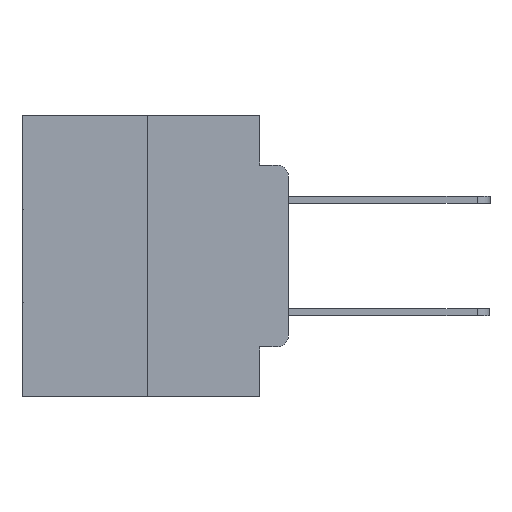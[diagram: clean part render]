
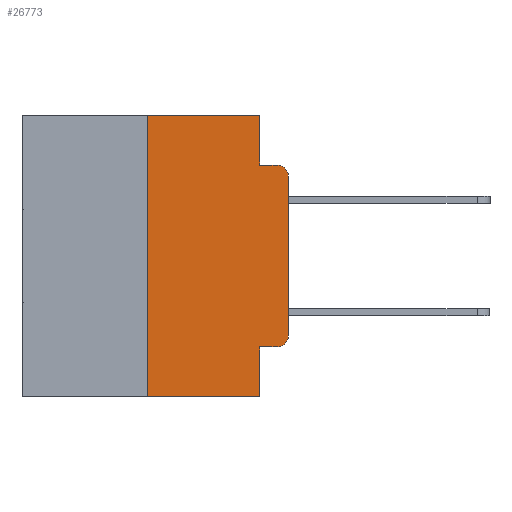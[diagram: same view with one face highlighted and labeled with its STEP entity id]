
A CAD part, left-side view. The second image highlights one B-rep face of the part: STEP entity #26773.
In plain terms, the highlighted planar face has unit normal (-1, 0, 0).
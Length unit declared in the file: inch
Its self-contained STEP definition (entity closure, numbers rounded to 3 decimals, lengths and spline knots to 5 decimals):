
#120 = CARTESIAN_POINT ( 'NONE',  ( 0., 0., -0.3915 ) ) ;
#135 = VECTOR ( 'NONE', #11315, 39.37008 ) ;
#243 = LINE ( 'NONE', #4427, #28844 ) ;
#1015 = EDGE_CURVE ( 'NONE', #17967, #27812, #6330, .T. ) ;
#1396 = DIRECTION ( 'NONE',  ( 0., -1., 0. ) ) ;
#1684 = DIRECTION ( 'NONE',  ( 0., 0., -1. ) ) ;
#2172 = CARTESIAN_POINT ( 'NONE',  ( 0., 0.473, -0.5 ) ) ;
#3479 = CARTESIAN_POINT ( 'NONE',  ( 0., 0.02, -0.1085 ) ) ;
#4118 = CARTESIAN_POINT ( 'NONE',  ( 0., 0.02, -0.4115 ) ) ;
#4162 = EDGE_CURVE ( 'NONE', #8578, #27812, #20606, .T. ) ;
#4427 = CARTESIAN_POINT ( 'NONE',  ( 0., 0.473, 0. ) ) ;
#4538 = VERTEX_POINT ( 'NONE', #120 ) ;
#4660 = ORIENTED_EDGE ( 'NONE', *, *, #19844, .F. ) ;
#4907 = CARTESIAN_POINT ( 'NONE',  ( 0., 0.051, 0. ) ) ;
#4984 = ORIENTED_EDGE ( 'NONE', *, *, #12306, .F. ) ;
#5018 = ORIENTED_EDGE ( 'NONE', *, *, #17750, .T. ) ;
#5283 = DIRECTION ( 'NONE',  ( 0., -1., 0. ) ) ;
#5596 = DIRECTION ( 'NONE',  ( 0., 0., -1. ) ) ;
#5604 = VECTOR ( 'NONE', #5283, 39.37008 ) ;
#5765 = DIRECTION ( 'NONE',  ( 0., 0., -1. ) ) ;
#6000 = LINE ( 'NONE', #21354, #22530 ) ;
#6330 = LINE ( 'NONE', #12679, #5604 ) ;
#6660 = AXIS2_PLACEMENT_3D ( 'NONE', #10825, #26447, #13093 ) ;
#6780 = VERTEX_POINT ( 'NONE', #12739 ) ;
#7205 = AXIS2_PLACEMENT_3D ( 'NONE', #3479, #19246, #5765 ) ;
#7244 = CIRCLE ( 'NONE', #8257, 0.02 ) ;
#7406 = CARTESIAN_POINT ( 'NONE',  ( 0., 0., 0. ) ) ;
#7486 = ORIENTED_EDGE ( 'NONE', *, *, #19971, .F. ) ;
#7498 = CARTESIAN_POINT ( 'NONE',  ( 0., 0.02, -0.3915 ) ) ;
#7599 = LINE ( 'NONE', #23391, #19578 ) ;
#7639 = EDGE_CURVE ( 'NONE', #6780, #13952, #7756, .T. ) ;
#7756 = LINE ( 'NONE', #2172, #135 ) ;
#8257 = AXIS2_PLACEMENT_3D ( 'NONE', #7498, #23208, #9790 ) ;
#8578 = VERTEX_POINT ( 'NONE', #15588 ) ;
#9292 = EDGE_CURVE ( 'NONE', #18075, #4538, #7244, .T. ) ;
#9790 = DIRECTION ( 'NONE',  ( 0., 0., -1. ) ) ;
#10809 = EDGE_CURVE ( 'NONE', #14582, #18075, #26771, .T. ) ;
#10825 = CARTESIAN_POINT ( 'NONE',  ( 0., 0.473, 0. ) ) ;
#11315 = DIRECTION ( 'NONE',  ( 0., -1., 0. ) ) ;
#12306 = EDGE_CURVE ( 'NONE', #14582, #13952, #6000, .T. ) ;
#12679 = CARTESIAN_POINT ( 'NONE',  ( 0., 0.051, -0.0885 ) ) ;
#12739 = CARTESIAN_POINT ( 'NONE',  ( 0., 0.25, -0.5 ) ) ;
#13093 = DIRECTION ( 'NONE',  ( 0., 0., -1. ) ) ;
#13952 = VERTEX_POINT ( 'NONE', #15835 ) ;
#14029 = VERTEX_POINT ( 'NONE', #4907 ) ;
#14582 = VERTEX_POINT ( 'NONE', #22897 ) ;
#14645 = CARTESIAN_POINT ( 'NONE',  ( 0., 0.25, 0. ) ) ;
#15230 = VECTOR ( 'NONE', #1684, 39.37008 ) ;
#15577 = ORIENTED_EDGE ( 'NONE', *, *, #7639, .T. ) ;
#15588 = CARTESIAN_POINT ( 'NONE',  ( 0., 0., -0.1085 ) ) ;
#15835 = CARTESIAN_POINT ( 'NONE',  ( 0., 0.051, -0.5 ) ) ;
#16306 = VECTOR ( 'NONE', #1396, 39.37008 ) ;
#16934 = ORIENTED_EDGE ( 'NONE', *, *, #9292, .T. ) ;
#17123 = VECTOR ( 'NONE', #20899, 39.37008 ) ;
#17297 = EDGE_LOOP ( 'NONE', ( #5018, #20174, #20883, #4660, #7486, #27461, #15577, #4984, #27433, #16934 ) ) ;
#17522 = CARTESIAN_POINT ( 'NONE',  ( 0., 0.051, 0. ) ) ;
#17750 = EDGE_CURVE ( 'NONE', #4538, #8578, #23086, .T. ) ;
#17967 = VERTEX_POINT ( 'NONE', #21678 ) ;
#18075 = VERTEX_POINT ( 'NONE', #4118 ) ;
#18311 = EDGE_CURVE ( 'NONE', #6780, #26038, #7599, .T. ) ;
#19246 = DIRECTION ( 'NONE',  ( -1., 0., 0. ) ) ;
#19425 = CARTESIAN_POINT ( 'NONE',  ( 0., 0.051, -0.4115 ) ) ;
#19578 = VECTOR ( 'NONE', #25588, 39.37008 ) ;
#19844 = EDGE_CURVE ( 'NONE', #14029, #17967, #27810, .T. ) ;
#19971 = EDGE_CURVE ( 'NONE', #26038, #14029, #243, .T. ) ;
#20174 = ORIENTED_EDGE ( 'NONE', *, *, #4162, .T. ) ;
#20606 = CIRCLE ( 'NONE', #7205, 0.02 ) ;
#20883 = ORIENTED_EDGE ( 'NONE', *, *, #1015, .F. ) ;
#20899 = DIRECTION ( 'NONE',  ( 0., 0., 1. ) ) ;
#21354 = CARTESIAN_POINT ( 'NONE',  ( 0., 0.051, 0. ) ) ;
#21678 = CARTESIAN_POINT ( 'NONE',  ( 0., 0.051, -0.0885 ) ) ;
#22012 = PLANE ( 'NONE',  #6660 ) ;
#22530 = VECTOR ( 'NONE', #5596, 39.37008 ) ;
#22897 = CARTESIAN_POINT ( 'NONE',  ( 0., 0.051, -0.4115 ) ) ;
#23086 = LINE ( 'NONE', #7406, #17123 ) ;
#23208 = DIRECTION ( 'NONE',  ( -1., 0., 0. ) ) ;
#23391 = CARTESIAN_POINT ( 'NONE',  ( 0., 0.25, 0. ) ) ;
#24641 = DIRECTION ( 'NONE',  ( 0., -1., 0. ) ) ;
#25588 = DIRECTION ( 'NONE',  ( 0., 0., 1. ) ) ;
#26038 = VERTEX_POINT ( 'NONE', #14645 ) ;
#26447 = DIRECTION ( 'NONE',  ( 1., 0., 0. ) ) ;
#26771 = LINE ( 'NONE', #19425, #16306 ) ;
#26773 = ADVANCED_FACE ( 'NONE', ( #26808 ), #22012, .F. ) ;
#26808 = FACE_OUTER_BOUND ( 'NONE', #17297, .T. ) ;
#27433 = ORIENTED_EDGE ( 'NONE', *, *, #10809, .T. ) ;
#27461 = ORIENTED_EDGE ( 'NONE', *, *, #18311, .F. ) ;
#27810 = LINE ( 'NONE', #17522, #15230 ) ;
#27812 = VERTEX_POINT ( 'NONE', #27936 ) ;
#27936 = CARTESIAN_POINT ( 'NONE',  ( 0., 0.02, -0.0885 ) ) ;
#28844 = VECTOR ( 'NONE', #24641, 39.37008 ) ;
